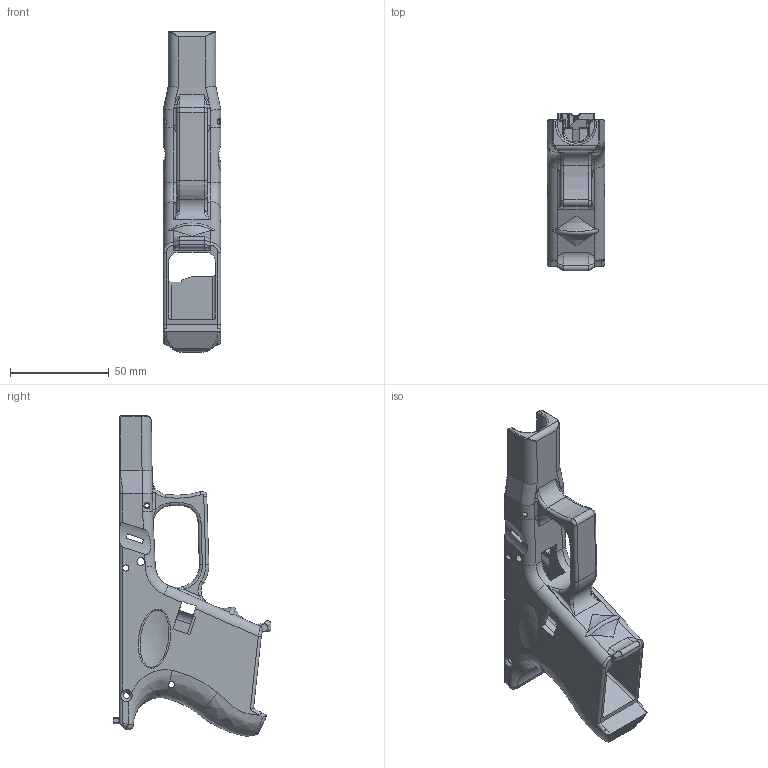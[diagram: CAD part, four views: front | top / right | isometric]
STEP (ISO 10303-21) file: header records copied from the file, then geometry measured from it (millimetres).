
FILE_DESCRIPTION(/* description */ (''),/* implementation_level */ '2;1');
FILE_NAME(/* name */ '4e6a65bf-8670-4999-b5e8-5b074afe6445.stp',/* time_stamp */ '2019-04-30T21:54:41-04:00',/* author */ (''),/* organization */ (''),/* preprocessor_version */ 'ST-DEVELOPER v18',/* originating_system */ 'Autodesk Translation Framework v8.2.0.1029',/* authorisation */ '');
FILE_SCHEMA (('AUTOMOTIVE_DESIGN { 1 0 10303 214 3 1 1 }'));
Length unit declared in the file: millimetre
Products named in the file (1): FusionComponent
Bounding box: 29.21 x 80.11 x 162.54 mm (x, y, z)
Volume: 74885.1 mm3; surface area: 37312.1 mm2
Topology: 1 solids, 1 shells, 451 faces, 1244 edges, 770 vertices
Faces by surface type: plane 160, cylinder 137, bspline 120, torus 30, sphere 2, cone 2
Full cylindrical faces by diameter (mm): 2.25 x2, 2.997 x2, 3 x2, 3.175 x2, 3.962 x2
Entity records: 35908 total; most frequent: CARTESIAN_POINT 25081, ORIENTED_EDGE 2472, DIRECTION 1994, EDGE_CURVE 1236, VERTEX_POINT 772, AXIS2_PLACEMENT_3D 710, LINE 574, VECTOR 574
